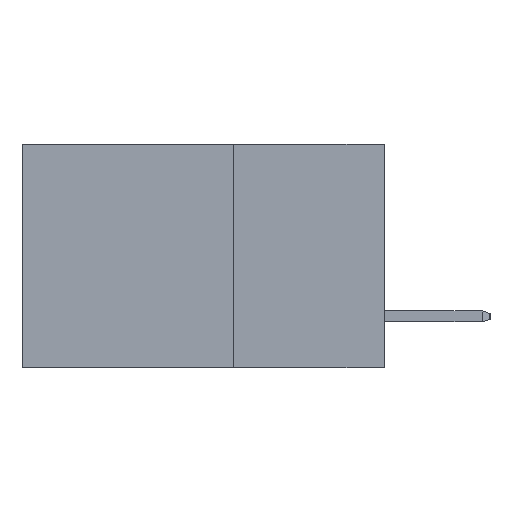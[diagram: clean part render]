
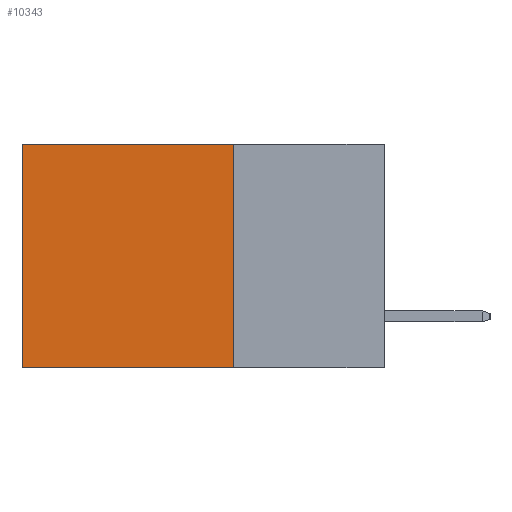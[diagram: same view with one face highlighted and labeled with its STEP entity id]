
A CAD part, left-side view. The second image highlights one B-rep face of the part: STEP entity #10343.
In plain terms, the highlighted planar face has unit normal (-1, 0, 0).
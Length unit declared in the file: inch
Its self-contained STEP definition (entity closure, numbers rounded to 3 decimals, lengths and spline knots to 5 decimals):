
#159 = EDGE_CURVE ( 'NONE', #5562, #17817, #15270, .T. ) ;
#369 = CARTESIAN_POINT ( 'NONE',  ( 0.2615, 0.25, -0.37 ) ) ;
#1239 = PLANE ( 'NONE',  #12881 ) ;
#2572 = VECTOR ( 'NONE', #16795, 39.37008 ) ;
#3059 = LINE ( 'NONE', #14064, #6614 ) ;
#3632 = DIRECTION ( 'NONE',  ( 0., 1., 0. ) ) ;
#5204 = ORIENTED_EDGE ( 'NONE', *, *, #7149, .T. ) ;
#5319 = CARTESIAN_POINT ( 'NONE',  ( 0.2615, 0.25, -0.37 ) ) ;
#5562 = VERTEX_POINT ( 'NONE', #17224 ) ;
#5574 = CARTESIAN_POINT ( 'NONE',  ( 0.2615, 0.6, 0. ) ) ;
#6077 = VERTEX_POINT ( 'NONE', #19414 ) ;
#6614 = VECTOR ( 'NONE', #3632, 39.37008 ) ;
#7149 = EDGE_CURVE ( 'NONE', #14818, #6077, #18371, .T. ) ;
#7356 = VECTOR ( 'NONE', #7867, 39.37008 ) ;
#7521 = CARTESIAN_POINT ( 'NONE',  ( 0.2615, 0.25, -0.37 ) ) ;
#7796 = EDGE_CURVE ( 'NONE', #5562, #14818, #3059, .T. ) ;
#7867 = DIRECTION ( 'NONE',  ( 0., 0., -1. ) ) ;
#9057 = DIRECTION ( 'NONE',  ( 0., 0., -1. ) ) ;
#9225 = ORIENTED_EDGE ( 'NONE', *, *, #159, .F. ) ;
#9600 = CARTESIAN_POINT ( 'NONE',  ( 0.2615, 0.25, -0.37 ) ) ;
#10343 = ADVANCED_FACE ( 'NONE', ( #13111 ), #1239, .F. ) ;
#10349 = EDGE_LOOP ( 'NONE', ( #5204, #16889, #9225, #15492 ) ) ;
#11210 = DIRECTION ( 'NONE',  ( 0., 1., 0. ) ) ;
#12881 = AXIS2_PLACEMENT_3D ( 'NONE', #7521, #17837, #9057 ) ;
#13111 = FACE_OUTER_BOUND ( 'NONE', #10349, .T. ) ;
#14064 = CARTESIAN_POINT ( 'NONE',  ( 0.2615, 0.25, 0. ) ) ;
#14818 = VERTEX_POINT ( 'NONE', #5574 ) ;
#15270 = LINE ( 'NONE', #5319, #7356 ) ;
#15492 = ORIENTED_EDGE ( 'NONE', *, *, #7796, .T. ) ;
#16667 = CARTESIAN_POINT ( 'NONE',  ( 0.2615, 0.6, -0.37 ) ) ;
#16795 = DIRECTION ( 'NONE',  ( 0., 0., -1. ) ) ;
#16889 = ORIENTED_EDGE ( 'NONE', *, *, #17866, .F. ) ;
#17224 = CARTESIAN_POINT ( 'NONE',  ( 0.2615, 0.25, 0. ) ) ;
#17817 = VERTEX_POINT ( 'NONE', #9600 ) ;
#17837 = DIRECTION ( 'NONE',  ( 1., 0., 0. ) ) ;
#17866 = EDGE_CURVE ( 'NONE', #17817, #6077, #18589, .T. ) ;
#18371 = LINE ( 'NONE', #16667, #2572 ) ;
#18589 = LINE ( 'NONE', #369, #19018 ) ;
#19018 = VECTOR ( 'NONE', #11210, 39.37008 ) ;
#19414 = CARTESIAN_POINT ( 'NONE',  ( 0.2615, 0.6, -0.37 ) ) ;
